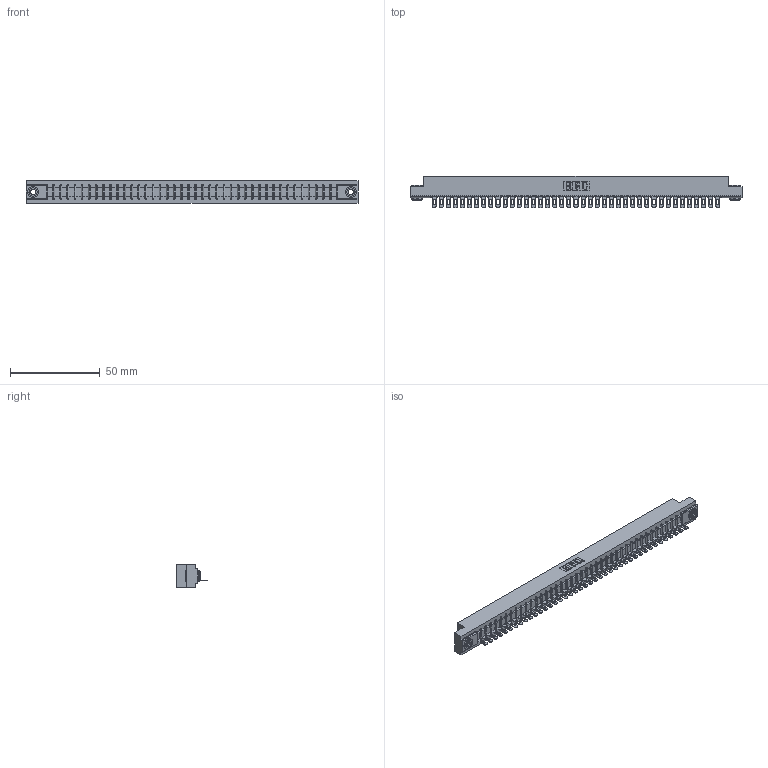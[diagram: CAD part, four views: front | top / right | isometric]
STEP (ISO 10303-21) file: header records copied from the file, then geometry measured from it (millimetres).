
FILE_DESCRIPTION (( 'STEP AP203' ), '1' );
FILE_NAME ('357-041-401-103.STEP', '2020-10-03T08:12:47', ( '' ), ( '' ), 'SwSTEP 2.0', 'SolidWorks 2020', '' );
FILE_SCHEMA (( 'CONFIG_CONTROL_DESIGN' ));
Length unit declared in the file: inch
Products named in the file (4): 307 Part_.156 Dia Mounting Holes; 345-250-002_345-250-002-102; 357-041-401-103; 307-290-002_501
Assembly tree (44 placements, depth 2):
  357-041-401-103
    307 Part_.156 Dia Mounting Holes
    307-290-002_501  x41
    345-250-002_345-250-002-102  x2
Bounding box: 185.47 x 17.42 x 12.7 mm (x, y, z)
Volume: 19877.3 mm3; surface area: 25497.1 mm2
Topology: 44 solids, 44 shells, 3328 faces, 10193 edges, 6678 vertices
Faces by surface type: plane 1898, cylinder 1338, sphere 84, cone 8
Entity records: 37131 total; most frequent: CARTESIAN_POINT 6241, ORIENTED_EDGE 6222, DIRECTION 6083, EDGE_CURVE 3111, LINE 2371, VECTOR 2371, VERTEX_POINT 2014, AXIS2_PLACEMENT_3D 1856
